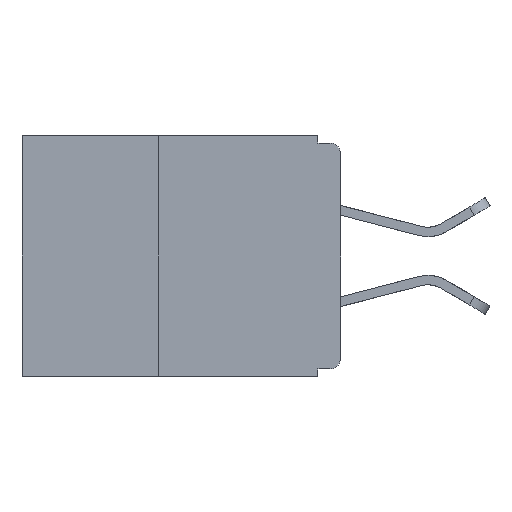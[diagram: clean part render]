
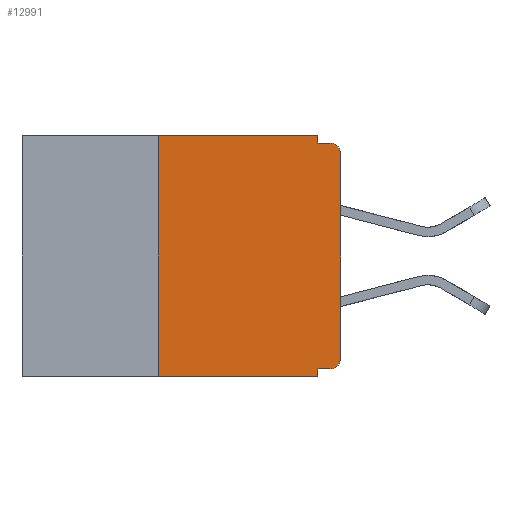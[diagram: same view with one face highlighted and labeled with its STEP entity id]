
A CAD part, left-side view. The second image highlights one B-rep face of the part: STEP entity #12991.
In plain terms, the highlighted planar face has unit normal (-1, 0, 0).
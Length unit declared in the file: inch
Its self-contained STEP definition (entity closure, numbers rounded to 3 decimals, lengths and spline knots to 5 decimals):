
#130 = ORIENTED_EDGE ( 'NONE', *, *, #10324, .T. ) ;
#282 = CARTESIAN_POINT ( 'NONE',  ( 0., 0., -0.025 ) ) ;
#565 = CARTESIAN_POINT ( 'NONE',  ( 0., 0.015, -0.025 ) ) ;
#584 = DIRECTION ( 'NONE',  ( 0., 0., -1. ) ) ;
#973 = CARTESIAN_POINT ( 'NONE',  ( 0., 0.015, -0.01 ) ) ;
#1245 = EDGE_CURVE ( 'NONE', #4016, #13139, #14273, .T. ) ;
#1758 = CARTESIAN_POINT ( 'NONE',  ( 0., 0.437, 0. ) ) ;
#1857 = DIRECTION ( 'NONE',  ( 0., 1., 0. ) ) ;
#2404 = DIRECTION ( 'NONE',  ( 0., 0., -1. ) ) ;
#2463 = LINE ( 'NONE', #18430, #6824 ) ;
#2464 = VECTOR ( 'NONE', #14474, 39.37008 ) ;
#3090 = FACE_OUTER_BOUND ( 'NONE', #7141, .T. ) ;
#3312 = AXIS2_PLACEMENT_3D ( 'NONE', #16516, #16428, #16200 ) ;
#4016 = VERTEX_POINT ( 'NONE', #9557 ) ;
#4095 = VECTOR ( 'NONE', #17266, 39.37008 ) ;
#4752 = EDGE_CURVE ( 'NONE', #15950, #20147, #18411, .T. ) ;
#4852 = ORIENTED_EDGE ( 'NONE', *, *, #12637, .F. ) ;
#4960 = CARTESIAN_POINT ( 'NONE',  ( 0., 0.25, 0. ) ) ;
#5144 = AXIS2_PLACEMENT_3D ( 'NONE', #6119, #11584, #584 ) ;
#5382 = ORIENTED_EDGE ( 'NONE', *, *, #4752, .T. ) ;
#5554 = VECTOR ( 'NONE', #23221, 39.37008 ) ;
#5721 = DIRECTION ( 'NONE',  ( 0., -1., 0. ) ) ;
#5802 = CARTESIAN_POINT ( 'NONE',  ( 0., 0.437, -0.33 ) ) ;
#5835 = ORIENTED_EDGE ( 'NONE', *, *, #1245, .F. ) ;
#5931 = CARTESIAN_POINT ( 'NONE',  ( 0., 0.25, -0.33 ) ) ;
#6083 = EDGE_CURVE ( 'NONE', #6093, #6930, #11712, .T. ) ;
#6093 = VERTEX_POINT ( 'NONE', #5931 ) ;
#6119 = CARTESIAN_POINT ( 'NONE',  ( 0., 0.437, 0. ) ) ;
#6824 = VECTOR ( 'NONE', #18131, 39.37008 ) ;
#6930 = VERTEX_POINT ( 'NONE', #18612 ) ;
#7141 = EDGE_LOOP ( 'NONE', ( #130, #10700, #5835, #4852, #15182, #23041, #18269, #11088, #11891, #5382 ) ) ;
#7376 = CARTESIAN_POINT ( 'NONE',  ( 0., 0., -0.32 ) ) ;
#7993 = EDGE_CURVE ( 'NONE', #6093, #15842, #2463, .T. ) ;
#8232 = VERTEX_POINT ( 'NONE', #10089 ) ;
#8498 = VERTEX_POINT ( 'NONE', #282 ) ;
#8687 = CARTESIAN_POINT ( 'NONE',  ( 0., 0.031, 0. ) ) ;
#8699 = EDGE_CURVE ( 'NONE', #8232, #6930, #22416, .T. ) ;
#9027 = LINE ( 'NONE', #7376, #22637 ) ;
#9332 = CARTESIAN_POINT ( 'NONE',  ( 0., 0., -0.01 ) ) ;
#9557 = CARTESIAN_POINT ( 'NONE',  ( 0., 0.031, -0.01 ) ) ;
#9741 = EDGE_CURVE ( 'NONE', #15950, #8232, #9027, .T. ) ;
#10089 = CARTESIAN_POINT ( 'NONE',  ( 0., 0.031, -0.32 ) ) ;
#10324 = EDGE_CURVE ( 'NONE', #20147, #8498, #15103, .T. ) ;
#10478 = DIRECTION ( 'NONE',  ( 0., 0., -1. ) ) ;
#10700 = ORIENTED_EDGE ( 'NONE', *, *, #11733, .T. ) ;
#11088 = ORIENTED_EDGE ( 'NONE', *, *, #8699, .F. ) ;
#11584 = DIRECTION ( 'NONE',  ( 1., 0., 0. ) ) ;
#11712 = LINE ( 'NONE', #5802, #14714 ) ;
#11733 = EDGE_CURVE ( 'NONE', #8498, #13139, #16955, .T. ) ;
#11891 = ORIENTED_EDGE ( 'NONE', *, *, #9741, .F. ) ;
#12637 = EDGE_CURVE ( 'NONE', #15361, #4016, #16351, .T. ) ;
#12991 = ADVANCED_FACE ( 'NONE', ( #3090 ), #22196, .F. ) ;
#13139 = VERTEX_POINT ( 'NONE', #973 ) ;
#13335 = DIRECTION ( 'NONE',  ( -1., 0., 0. ) ) ;
#14249 = CARTESIAN_POINT ( 'NONE',  ( 0., 0.015, -0.32 ) ) ;
#14273 = LINE ( 'NONE', #9332, #4095 ) ;
#14474 = DIRECTION ( 'NONE',  ( 0., -1., 0. ) ) ;
#14614 = AXIS2_PLACEMENT_3D ( 'NONE', #565, #13335, #2404 ) ;
#14714 = VECTOR ( 'NONE', #5721, 39.37008 ) ;
#15103 = LINE ( 'NONE', #23150, #5554 ) ;
#15182 = ORIENTED_EDGE ( 'NONE', *, *, #19779, .F. ) ;
#15361 = VERTEX_POINT ( 'NONE', #22950 ) ;
#15818 = VECTOR ( 'NONE', #10478, 39.37008 ) ;
#15842 = VERTEX_POINT ( 'NONE', #4960 ) ;
#15950 = VERTEX_POINT ( 'NONE', #14249 ) ;
#16200 = DIRECTION ( 'NONE',  ( 0., 0., -1. ) ) ;
#16309 = CARTESIAN_POINT ( 'NONE',  ( 0., 0., -0.305 ) ) ;
#16351 = LINE ( 'NONE', #8687, #15818 ) ;
#16428 = DIRECTION ( 'NONE',  ( -1., 0., 0. ) ) ;
#16454 = CARTESIAN_POINT ( 'NONE',  ( 0., 0.031, -0.33 ) ) ;
#16516 = CARTESIAN_POINT ( 'NONE',  ( 0., 0.015, -0.305 ) ) ;
#16955 = CIRCLE ( 'NONE', #14614, 0.015 ) ;
#17266 = DIRECTION ( 'NONE',  ( 0., -1., 0. ) ) ;
#17680 = VECTOR ( 'NONE', #18270, 39.37008 ) ;
#18131 = DIRECTION ( 'NONE',  ( 0., 0., 1. ) ) ;
#18269 = ORIENTED_EDGE ( 'NONE', *, *, #6083, .T. ) ;
#18270 = DIRECTION ( 'NONE',  ( 0., 0., -1. ) ) ;
#18411 = CIRCLE ( 'NONE', #3312, 0.015 ) ;
#18430 = CARTESIAN_POINT ( 'NONE',  ( 0., 0.25, -0.33 ) ) ;
#18612 = CARTESIAN_POINT ( 'NONE',  ( 0., 0.031, -0.33 ) ) ;
#19779 = EDGE_CURVE ( 'NONE', #15842, #15361, #21088, .T. ) ;
#20147 = VERTEX_POINT ( 'NONE', #16309 ) ;
#21088 = LINE ( 'NONE', #1758, #2464 ) ;
#22196 = PLANE ( 'NONE',  #5144 ) ;
#22416 = LINE ( 'NONE', #16454, #17680 ) ;
#22637 = VECTOR ( 'NONE', #1857, 39.37008 ) ;
#22950 = CARTESIAN_POINT ( 'NONE',  ( 0., 0.031, 0. ) ) ;
#23041 = ORIENTED_EDGE ( 'NONE', *, *, #7993, .F. ) ;
#23150 = CARTESIAN_POINT ( 'NONE',  ( 0., 0., 0. ) ) ;
#23221 = DIRECTION ( 'NONE',  ( 0., 0., 1. ) ) ;
